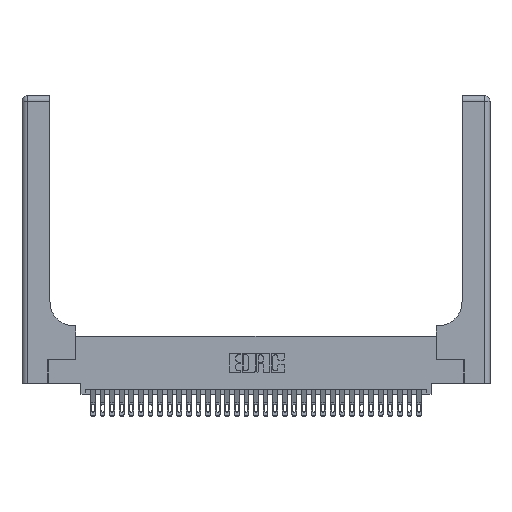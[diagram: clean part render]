
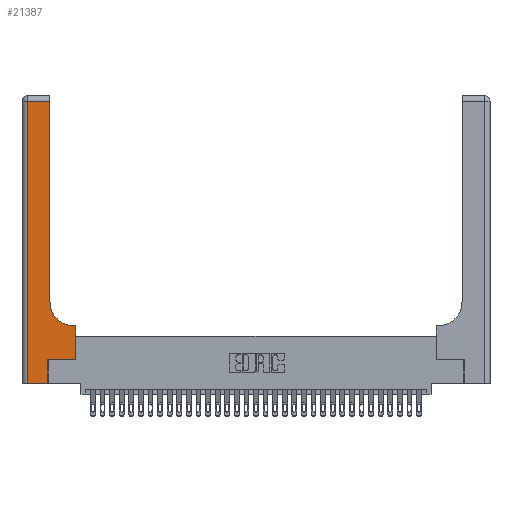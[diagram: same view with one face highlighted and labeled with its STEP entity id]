
A CAD part, top view. The second image highlights one B-rep face of the part: STEP entity #21387.
In plain terms, the highlighted planar face has unit normal (0, 0, 1).
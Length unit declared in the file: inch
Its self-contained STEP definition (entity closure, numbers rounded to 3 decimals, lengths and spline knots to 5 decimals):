
#152 = EDGE_CURVE ( 'NONE', #8781, #20509, #743, .T. ) ;
#743 = LINE ( 'NONE', #20686, #28786 ) ;
#1135 = EDGE_CURVE ( 'NONE', #24488, #8781, #13040, .T. ) ;
#2171 = VERTEX_POINT ( 'NONE', #18246 ) ;
#2198 = ORIENTED_EDGE ( 'NONE', *, *, #11014, .T. ) ;
#2534 = LINE ( 'NONE', #9869, #9557 ) ;
#2561 = ORIENTED_EDGE ( 'NONE', *, *, #4567, .T. ) ;
#2901 = CARTESIAN_POINT ( 'NONE',  ( 0.2915, 0.6, 0.37 ) ) ;
#3010 = AXIS2_PLACEMENT_3D ( 'NONE', #21987, #6181, #24644 ) ;
#4567 = EDGE_CURVE ( 'NONE', #4689, #9414, #17750, .T. ) ;
#4689 = VERTEX_POINT ( 'NONE', #26971 ) ;
#4887 = DIRECTION ( 'NONE',  ( 0., 1., 0. ) ) ;
#5027 = ORIENTED_EDGE ( 'NONE', *, *, #18234, .T. ) ;
#5323 = VECTOR ( 'NONE', #14956, 39.37008 ) ;
#6006 = VECTOR ( 'NONE', #14970, 39.37008 ) ;
#6146 = LINE ( 'NONE', #28100, #5323 ) ;
#6181 = DIRECTION ( 'NONE',  ( 0., 0., -1. ) ) ;
#6694 = ORIENTED_EDGE ( 'NONE', *, *, #26755, .T. ) ;
#6847 = LINE ( 'NONE', #25561, #6006 ) ;
#6996 = DIRECTION ( 'NONE',  ( 0., 1., 0. ) ) ;
#7503 = ORIENTED_EDGE ( 'NONE', *, *, #16827, .T. ) ;
#8781 = VERTEX_POINT ( 'NONE', #19721 ) ;
#9414 = VERTEX_POINT ( 'NONE', #11893 ) ;
#9557 = VECTOR ( 'NONE', #12527, 39.37008 ) ;
#9565 = PLANE ( 'NONE',  #28806 ) ;
#9869 = CARTESIAN_POINT ( 'NONE',  ( 0.269, 0.25, 0.37 ) ) ;
#10017 = VERTEX_POINT ( 'NONE', #32664 ) ;
#11014 = EDGE_CURVE ( 'NONE', #12396, #24488, #18445, .T. ) ;
#11893 = CARTESIAN_POINT ( 'NONE',  ( 0.06, 0., 0.37 ) ) ;
#12097 = EDGE_CURVE ( 'NONE', #20509, #4689, #6847, .T. ) ;
#12396 = VERTEX_POINT ( 'NONE', #18959 ) ;
#12527 = DIRECTION ( 'NONE',  ( 1., 0., 0. ) ) ;
#12715 = VERTEX_POINT ( 'NONE', #25392 ) ;
#13040 = CIRCLE ( 'NONE', #3010, 0.25 ) ;
#13246 = CARTESIAN_POINT ( 'NONE',  ( 0.06, 3., 0.37 ) ) ;
#13654 = LINE ( 'NONE', #25482, #19842 ) ;
#14883 = DIRECTION ( 'NONE',  ( -1., 0., 0. ) ) ;
#14956 = DIRECTION ( 'NONE',  ( 1., 0., 0. ) ) ;
#14970 = DIRECTION ( 'NONE',  ( -1., 0., 0. ) ) ;
#16827 = EDGE_CURVE ( 'NONE', #10017, #12715, #13654, .T. ) ;
#17482 = DIRECTION ( 'NONE',  ( 0., 1., 0. ) ) ;
#17750 = LINE ( 'NONE', #13246, #30902 ) ;
#18234 = EDGE_CURVE ( 'NONE', #9414, #10017, #6146, .T. ) ;
#18246 = CARTESIAN_POINT ( 'NONE',  ( 0.5585, 0.25, 0.37 ) ) ;
#18445 = LINE ( 'NONE', #2901, #31597 ) ;
#18692 = DIRECTION ( 'NONE',  ( -1., 0., 0. ) ) ;
#18959 = CARTESIAN_POINT ( 'NONE',  ( 0.5585, 0.6, 0.37 ) ) ;
#19721 = CARTESIAN_POINT ( 'NONE',  ( 0.2915, 0.85, 0.37 ) ) ;
#19842 = VECTOR ( 'NONE', #6996, 39.37008 ) ;
#20509 = VERTEX_POINT ( 'NONE', #32266 ) ;
#20686 = CARTESIAN_POINT ( 'NONE',  ( 0.2915, 3., 0.37 ) ) ;
#21120 = EDGE_LOOP ( 'NONE', ( #23175, #28954, #2561, #5027, #7503, #28983, #6694, #2198, #33500 ) ) ;
#21387 = ADVANCED_FACE ( 'NONE', ( #27229 ), #9565, .F. ) ;
#21987 = CARTESIAN_POINT ( 'NONE',  ( 0.5415, 0.85, 0.37 ) ) ;
#22246 = VECTOR ( 'NONE', #17482, 39.37008 ) ;
#22661 = CARTESIAN_POINT ( 'NONE',  ( 0.5585, 0.25, 0.37 ) ) ;
#23175 = ORIENTED_EDGE ( 'NONE', *, *, #152, .T. ) ;
#24488 = VERTEX_POINT ( 'NONE', #29288 ) ;
#24644 = DIRECTION ( 'NONE',  ( 1., 0., 0. ) ) ;
#25392 = CARTESIAN_POINT ( 'NONE',  ( 0.269, 0.25, 0.37 ) ) ;
#25482 = CARTESIAN_POINT ( 'NONE',  ( 0.269, 0., 0.37 ) ) ;
#25557 = EDGE_CURVE ( 'NONE', #12715, #2171, #2534, .T. ) ;
#25561 = CARTESIAN_POINT ( 'NONE',  ( 0., 2.94, 0.37 ) ) ;
#26755 = EDGE_CURVE ( 'NONE', #2171, #12396, #29255, .T. ) ;
#26971 = CARTESIAN_POINT ( 'NONE',  ( 0.06, 2.94, 0.37 ) ) ;
#27229 = FACE_OUTER_BOUND ( 'NONE', #21120, .T. ) ;
#28013 = CARTESIAN_POINT ( 'NONE',  ( 0., 3., 0.37 ) ) ;
#28100 = CARTESIAN_POINT ( 'NONE',  ( 0., 0., 0.37 ) ) ;
#28786 = VECTOR ( 'NONE', #4887, 39.37008 ) ;
#28806 = AXIS2_PLACEMENT_3D ( 'NONE', #28013, #30616, #14883 ) ;
#28954 = ORIENTED_EDGE ( 'NONE', *, *, #12097, .T. ) ;
#28983 = ORIENTED_EDGE ( 'NONE', *, *, #25557, .T. ) ;
#29255 = LINE ( 'NONE', #22661, #22246 ) ;
#29288 = CARTESIAN_POINT ( 'NONE',  ( 0.5415, 0.6, 0.37 ) ) ;
#30616 = DIRECTION ( 'NONE',  ( 0., 0., -1. ) ) ;
#30902 = VECTOR ( 'NONE', #31536, 39.37008 ) ;
#31536 = DIRECTION ( 'NONE',  ( 0., -1., 0. ) ) ;
#31597 = VECTOR ( 'NONE', #18692, 39.37008 ) ;
#32266 = CARTESIAN_POINT ( 'NONE',  ( 0.2915, 2.94, 0.37 ) ) ;
#32664 = CARTESIAN_POINT ( 'NONE',  ( 0.269, 0., 0.37 ) ) ;
#33500 = ORIENTED_EDGE ( 'NONE', *, *, #1135, .T. ) ;
